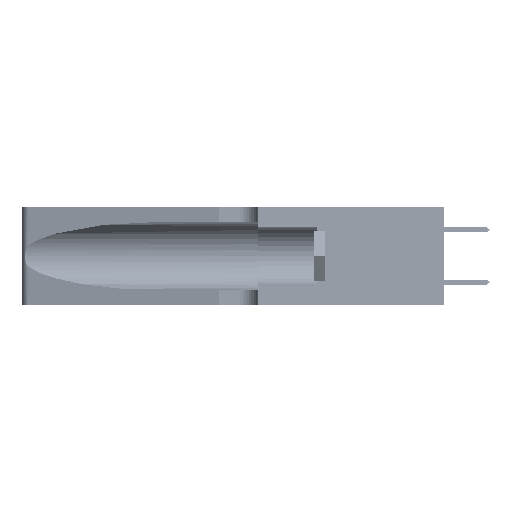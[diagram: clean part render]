
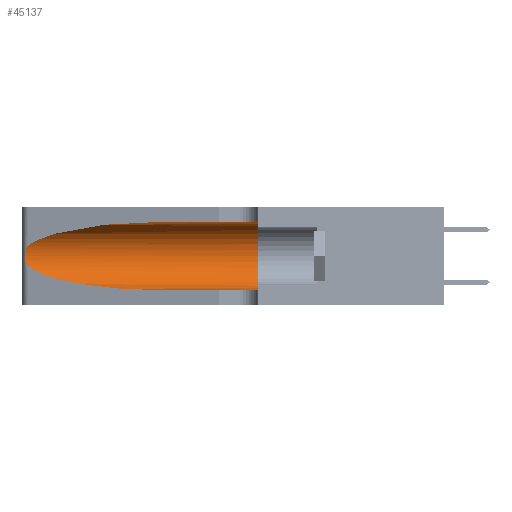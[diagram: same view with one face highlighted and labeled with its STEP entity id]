
A CAD part, left-side view. The second image highlights one B-rep face of the part: STEP entity #45137.
In plain terms, the highlighted cylindrical face has radius 3.308 mm (diameter 6.617 mm), a partial arc.
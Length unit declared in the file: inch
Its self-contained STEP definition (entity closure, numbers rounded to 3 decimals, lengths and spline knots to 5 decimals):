
#628 = ORIENTED_EDGE ( 'NONE', *, *, #47392, .T. ) ;
#1541 = CARTESIAN_POINT ( 'NONE',  ( 0.1305, 1.61858, 0.185 ) ) ;
#1984 = CARTESIAN_POINT ( 'NONE',  ( 0.25487, 1.22718, 0.22369 ) ) ;
#2618 = EDGE_CURVE ( 'NONE', #38494, #35016, #5139, .T. ) ;
#2805 = CARTESIAN_POINT ( 'NONE',  ( 0.26075, 1.23896, 0.19203 ) ) ;
#4543 =( BOUNDED_CURVE ( )  B_SPLINE_CURVE ( 3, ( #33984, #41480, #44927, #4547 ),
 .UNSPECIFIED., .F., .F. ) 
 B_SPLINE_CURVE_WITH_KNOTS ( ( 4, 4 ),
 ( 1.5708, 2.84003 ),
 .UNSPECIFIED. ) 
 CURVE ( )  GEOMETRIC_REPRESENTATION_ITEM ( )  RATIONAL_B_SPLINE_CURVE ( ( 1., 0.87, 0.87, 1. ) ) 
 REPRESENTATION_ITEM ( '' )  );
#4547 = CARTESIAN_POINT ( 'NONE',  ( 0.25487, 1.22718, 0.22369 ) ) ;
#5107 = DIRECTION ( 'NONE',  ( 0., -1., 0. ) ) ;
#5139 =( BOUNDED_CURVE ( )  B_SPLINE_CURVE ( 3, ( #34864, #37969, #12442, #38633 ),
 .UNSPECIFIED., .F., .T. ) 
 B_SPLINE_CURVE_WITH_KNOTS ( ( 4, 4 ),
 ( 3.44316, 4.71239 ),
 .UNSPECIFIED. ) 
 CURVE ( )  GEOMETRIC_REPRESENTATION_ITEM ( )  RATIONAL_B_SPLINE_CURVE ( ( 1., 0.87, 0.87, 1. ) ) 
 REPRESENTATION_ITEM ( '' )  );
#6556 = CARTESIAN_POINT ( 'NONE',  ( 0.26075, 1.23896, 0.178 ) ) ;
#8392 = CARTESIAN_POINT ( 'NONE',  ( 0.1305, 0.72297, 0.05475 ) ) ;
#9037 = CARTESIAN_POINT ( 'NONE',  ( 0.1305, 1.61858, 0.05475 ) ) ;
#9594 = VERTEX_POINT ( 'NONE', #25197 ) ;
#10299 = CARTESIAN_POINT ( 'NONE',  ( 0.25555, 1.22993, 0.14849 ) ) ;
#11885 = VECTOR ( 'NONE', #5107, 39.37008 ) ;
#12442 = CARTESIAN_POINT ( 'NONE',  ( 0.18966, 0.96281, 0.05475 ) ) ;
#13546 = CARTESIAN_POINT ( 'NONE',  ( 0.1305, 0.35, 0.185 ) ) ;
#13920 = CARTESIAN_POINT ( 'NONE',  ( 0.25555, 1.22994, 0.2215 ) ) ;
#14853 = DIRECTION ( 'NONE',  ( 0., -1., 0. ) ) ;
#15267 = EDGE_CURVE ( 'NONE', #40367, #9594, #30853, .T. ) ;
#16430 = ORIENTED_EDGE ( 'NONE', *, *, #34103, .F. ) ;
#20301 = EDGE_CURVE ( 'NONE', #40367, #34076, #4543, .T. ) ;
#21085 = ORIENTED_EDGE ( 'NONE', *, *, #20301, .T. ) ;
#21607 = CARTESIAN_POINT ( 'NONE',  ( 0.25787, 1.23484, 0.2124 ) ) ;
#21957 = ORIENTED_EDGE ( 'NONE', *, *, #15267, .F. ) ;
#25197 = CARTESIAN_POINT ( 'NONE',  ( 0.1305, 0.35, 0.31525 ) ) ;
#26086 = FACE_OUTER_BOUND ( 'NONE', #32284, .T. ) ;
#26707 = CYLINDRICAL_SURFACE ( 'NONE', #44717, 0.13025 ) ;
#27203 = DIRECTION ( 'NONE',  ( 0., -1., 0. ) ) ;
#28640 = CARTESIAN_POINT ( 'NONE',  ( 0.1305, 0.72297, 0.31525 ) ) ;
#28807 = CARTESIAN_POINT ( 'NONE',  ( 0.25854, 1.2359, 0.20912 ) ) ;
#28966 = CARTESIAN_POINT ( 'NONE',  ( 0.25487, 1.22718, 0.22369 ) ) ;
#29135 = B_SPLINE_CURVE_WITH_KNOTS ( 'NONE', 3,
 ( #28966, #13920, #40216, #21607, #28807, #36970, #2805, #6556, #47720, #47411, #36816, #32709, #10299, #36352 ),
 .UNSPECIFIED., .F., .F.,
 ( 4, 2, 2, 2, 2, 2, 4 ),
 ( 0., 0.00027, 0.00053, 0.00107, 0.0016, 0.00187, 0.00214 ),
 .UNSPECIFIED. ) ;
#30853 = LINE ( 'NONE', #44584, #33747 ) ;
#31270 = DIRECTION ( 'NONE',  ( 0., 0., -1. ) ) ;
#31587 = VERTEX_POINT ( 'NONE', #36145 ) ;
#32132 = CIRCLE ( 'NONE', #37230, 0.13025 ) ;
#32284 = EDGE_LOOP ( 'NONE', ( #21085, #38994, #47328, #628, #16430, #21957 ) ) ;
#32709 = CARTESIAN_POINT ( 'NONE',  ( 0.25639, 1.23186, 0.15144 ) ) ;
#33747 = VECTOR ( 'NONE', #14853, 39.37008 ) ;
#33984 = CARTESIAN_POINT ( 'NONE',  ( 0.1305, 0.72297, 0.31525 ) ) ;
#34076 = VERTEX_POINT ( 'NONE', #1984 ) ;
#34103 = EDGE_CURVE ( 'NONE', #9594, #31587, #32132, .T. ) ;
#34864 = CARTESIAN_POINT ( 'NONE',  ( 0.25487, 1.22718, 0.14631 ) ) ;
#35016 = VERTEX_POINT ( 'NONE', #8392 ) ;
#36145 = CARTESIAN_POINT ( 'NONE',  ( 0.1305, 0.35, 0.05475 ) ) ;
#36163 = CARTESIAN_POINT ( 'NONE',  ( 0.25487, 1.22718, 0.14631 ) ) ;
#36352 = CARTESIAN_POINT ( 'NONE',  ( 0.25487, 1.22718, 0.14631 ) ) ;
#36514 = LINE ( 'NONE', #9037, #11885 ) ;
#36816 = CARTESIAN_POINT ( 'NONE',  ( 0.25789, 1.23486, 0.15765 ) ) ;
#36970 = CARTESIAN_POINT ( 'NONE',  ( 0.26018, 1.23835, 0.19895 ) ) ;
#37230 = AXIS2_PLACEMENT_3D ( 'NONE', #13546, #43439, #39070 ) ;
#37969 = CARTESIAN_POINT ( 'NONE',  ( 0.2373, 1.15595, 0.08982 ) ) ;
#38494 = VERTEX_POINT ( 'NONE', #36163 ) ;
#38633 = CARTESIAN_POINT ( 'NONE',  ( 0.1305, 0.72297, 0.05475 ) ) ;
#38994 = ORIENTED_EDGE ( 'NONE', *, *, #40401, .T. ) ;
#39070 = DIRECTION ( 'NONE',  ( 0., 0., 1. ) ) ;
#40216 = CARTESIAN_POINT ( 'NONE',  ( 0.25639, 1.23184, 0.21858 ) ) ;
#40367 = VERTEX_POINT ( 'NONE', #28640 ) ;
#40401 = EDGE_CURVE ( 'NONE', #34076, #38494, #29135, .T. ) ;
#41480 = CARTESIAN_POINT ( 'NONE',  ( 0.18966, 0.96281, 0.31525 ) ) ;
#43439 = DIRECTION ( 'NONE',  ( 0., 1., 0. ) ) ;
#44584 = CARTESIAN_POINT ( 'NONE',  ( 0.1305, 1.61858, 0.31525 ) ) ;
#44717 = AXIS2_PLACEMENT_3D ( 'NONE', #1541, #27203, #31270 ) ;
#44927 = CARTESIAN_POINT ( 'NONE',  ( 0.2373, 1.15595, 0.28018 ) ) ;
#45137 = ADVANCED_FACE ( 'NONE', ( #26086 ), #26707, .F. ) ;
#47328 = ORIENTED_EDGE ( 'NONE', *, *, #2618, .T. ) ;
#47392 = EDGE_CURVE ( 'NONE', #35016, #31587, #36514, .T. ) ;
#47411 = CARTESIAN_POINT ( 'NONE',  ( 0.25856, 1.23593, 0.16098 ) ) ;
#47720 = CARTESIAN_POINT ( 'NONE',  ( 0.26017, 1.23833, 0.17102 ) ) ;
